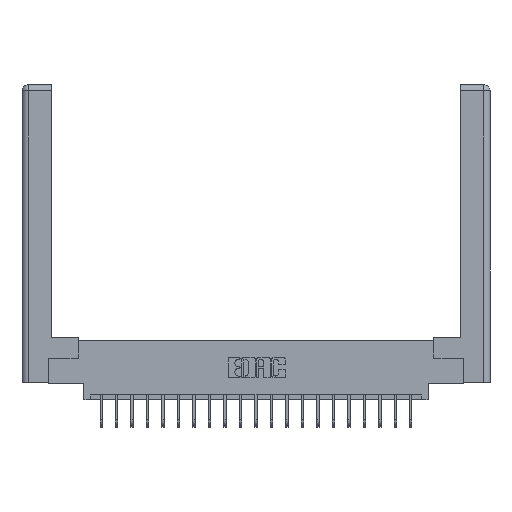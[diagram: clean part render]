
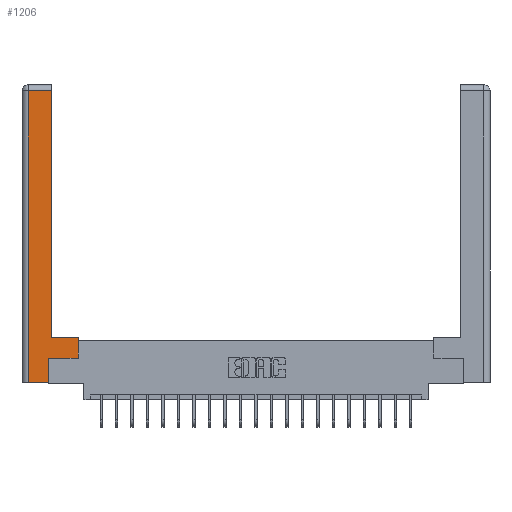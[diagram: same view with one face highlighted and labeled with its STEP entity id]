
A CAD part, top view. The second image highlights one B-rep face of the part: STEP entity #1206.
In plain terms, the highlighted planar face has unit normal (0, 0, 1).
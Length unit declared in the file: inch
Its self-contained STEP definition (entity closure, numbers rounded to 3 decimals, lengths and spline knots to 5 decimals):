
#192 = VERTEX_POINT ( 'NONE', #3249 ) ;
#334 = ORIENTED_EDGE ( 'NONE', *, *, #2085, .T. ) ;
#925 = EDGE_CURVE ( 'NONE', #6000, #14872, #17818, .T. ) ;
#1206 = ADVANCED_FACE ( 'NONE', ( #14370 ), #4614, .F. ) ;
#2085 = EDGE_CURVE ( 'NONE', #7226, #192, #15631, .T. ) ;
#3249 = CARTESIAN_POINT ( 'NONE',  ( 0.295, 2.94, 0. ) ) ;
#3317 = DIRECTION ( 'NONE',  ( 0., 1., 0. ) ) ;
#3556 = EDGE_CURVE ( 'NONE', #5076, #7757, #13254, .T. ) ;
#4237 = LINE ( 'NONE', #13680, #5677 ) ;
#4614 = PLANE ( 'NONE',  #10919 ) ;
#4684 = CARTESIAN_POINT ( 'NONE',  ( 0.565, 0.45, 0. ) ) ;
#5076 = VERTEX_POINT ( 'NONE', #8740 ) ;
#5677 = VECTOR ( 'NONE', #3317, 39.37008 ) ;
#6000 = VERTEX_POINT ( 'NONE', #12537 ) ;
#6174 = DIRECTION ( 'NONE',  ( 0., 1., 0. ) ) ;
#6803 = VERTEX_POINT ( 'NONE', #4684 ) ;
#7200 = CARTESIAN_POINT ( 'NONE',  ( 0.295, 3., 0. ) ) ;
#7226 = VERTEX_POINT ( 'NONE', #20347 ) ;
#7656 = CARTESIAN_POINT ( 'NONE',  ( 0.295, 0.45, 0. ) ) ;
#7757 = VERTEX_POINT ( 'NONE', #18811 ) ;
#7888 = CARTESIAN_POINT ( 'NONE',  ( 0.265, 0., 0. ) ) ;
#8352 = DIRECTION ( 'NONE',  ( 0., 0., -1. ) ) ;
#8715 = CARTESIAN_POINT ( 'NONE',  ( 0.265, 0., 0. ) ) ;
#8740 = CARTESIAN_POINT ( 'NONE',  ( 0.0615, 2.94, 0. ) ) ;
#8957 = VECTOR ( 'NONE', #22668, 39.37008 ) ;
#9703 = ORIENTED_EDGE ( 'NONE', *, *, #925, .T. ) ;
#9807 = EDGE_CURVE ( 'NONE', #22765, #6000, #13516, .T. ) ;
#9856 = LINE ( 'NONE', #8715, #21237 ) ;
#9989 = ORIENTED_EDGE ( 'NONE', *, *, #14066, .T. ) ;
#10238 = EDGE_LOOP ( 'NONE', ( #334, #9989, #14838, #18144, #20790, #9703, #21125, #13984 ) ) ;
#10662 = VECTOR ( 'NONE', #15536, 39.37008 ) ;
#10763 = VECTOR ( 'NONE', #23330, 39.37008 ) ;
#10776 = CARTESIAN_POINT ( 'NONE',  ( 0.0615, 0., 0. ) ) ;
#10919 = AXIS2_PLACEMENT_3D ( 'NONE', #19254, #8352, #22962 ) ;
#10982 = VECTOR ( 'NONE', #15906, 39.37008 ) ;
#12505 = DIRECTION ( 'NONE',  ( -1., 0., 0. ) ) ;
#12537 = CARTESIAN_POINT ( 'NONE',  ( 0.265, 0.245, 0. ) ) ;
#12916 = CARTESIAN_POINT ( 'NONE',  ( 0.265, 0.245, 0. ) ) ;
#13254 = LINE ( 'NONE', #10776, #10982 ) ;
#13325 = EDGE_CURVE ( 'NONE', #14872, #6803, #4237, .T. ) ;
#13516 = LINE ( 'NONE', #12916, #14401 ) ;
#13680 = CARTESIAN_POINT ( 'NONE',  ( 0.565, 0.45, 0. ) ) ;
#13905 = LINE ( 'NONE', #17614, #22418 ) ;
#13984 = ORIENTED_EDGE ( 'NONE', *, *, #22637, .T. ) ;
#14066 = EDGE_CURVE ( 'NONE', #192, #5076, #13905, .T. ) ;
#14370 = FACE_OUTER_BOUND ( 'NONE', #10238, .T. ) ;
#14401 = VECTOR ( 'NONE', #6174, 39.37008 ) ;
#14838 = ORIENTED_EDGE ( 'NONE', *, *, #3556, .T. ) ;
#14872 = VERTEX_POINT ( 'NONE', #22798 ) ;
#15536 = DIRECTION ( 'NONE',  ( 1., 0., 0. ) ) ;
#15631 = LINE ( 'NONE', #7200, #10763 ) ;
#15906 = DIRECTION ( 'NONE',  ( 0., -1., 0. ) ) ;
#16103 = EDGE_CURVE ( 'NONE', #7757, #22765, #9856, .T. ) ;
#17614 = CARTESIAN_POINT ( 'NONE',  ( 0.0615, 2.94, 0. ) ) ;
#17818 = LINE ( 'NONE', #18367, #10662 ) ;
#18144 = ORIENTED_EDGE ( 'NONE', *, *, #16103, .T. ) ;
#18367 = CARTESIAN_POINT ( 'NONE',  ( 0.565, 0.245, 0. ) ) ;
#18811 = CARTESIAN_POINT ( 'NONE',  ( 0.0615, 0., 0. ) ) ;
#19254 = CARTESIAN_POINT ( 'NONE',  ( 0., 0., 0. ) ) ;
#20347 = CARTESIAN_POINT ( 'NONE',  ( 0.295, 0.45, 0. ) ) ;
#20790 = ORIENTED_EDGE ( 'NONE', *, *, #9807, .T. ) ;
#21125 = ORIENTED_EDGE ( 'NONE', *, *, #13325, .T. ) ;
#21237 = VECTOR ( 'NONE', #21427, 39.37008 ) ;
#21427 = DIRECTION ( 'NONE',  ( 1., 0., 0. ) ) ;
#22418 = VECTOR ( 'NONE', #12505, 39.37008 ) ;
#22637 = EDGE_CURVE ( 'NONE', #6803, #7226, #22876, .T. ) ;
#22668 = DIRECTION ( 'NONE',  ( -1., 0., 0. ) ) ;
#22765 = VERTEX_POINT ( 'NONE', #7888 ) ;
#22798 = CARTESIAN_POINT ( 'NONE',  ( 0.565, 0.245, 0. ) ) ;
#22876 = LINE ( 'NONE', #7656, #8957 ) ;
#22962 = DIRECTION ( 'NONE',  ( -1., 0., 0. ) ) ;
#23330 = DIRECTION ( 'NONE',  ( 0., 1., 0. ) ) ;
